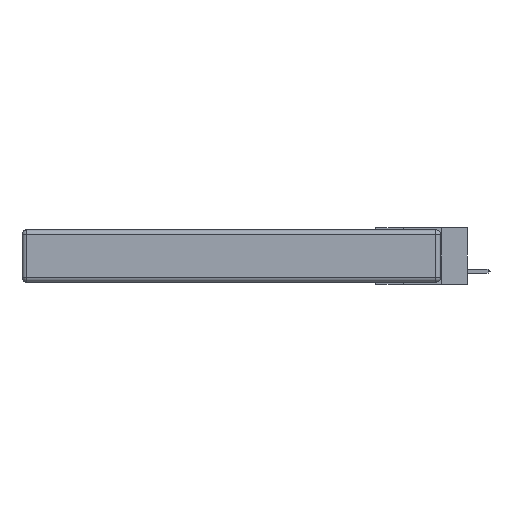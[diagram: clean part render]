
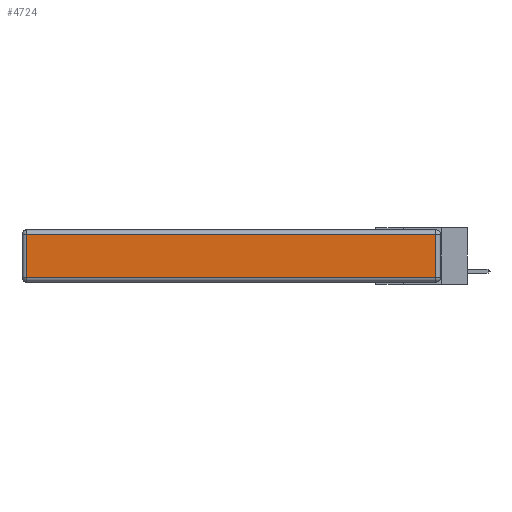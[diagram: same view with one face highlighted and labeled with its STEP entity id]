
A CAD part, left-side view. The second image highlights one B-rep face of the part: STEP entity #4724.
In plain terms, the highlighted planar face has unit normal (-1, 0, 0).
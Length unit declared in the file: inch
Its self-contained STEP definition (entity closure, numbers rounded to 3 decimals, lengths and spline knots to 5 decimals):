
#19 = CARTESIAN_POINT ( 'NONE',  ( 0., 2.72, -0.343 ) ) ;
#664 = CARTESIAN_POINT ( 'NONE',  ( 0., 0., -0.313 ) ) ;
#1249 = DIRECTION ( 'NONE',  ( 0., 0., 1. ) ) ;
#1866 = DIRECTION ( 'NONE',  ( 0., 1., 0. ) ) ;
#1868 = ORIENTED_EDGE ( 'NONE', *, *, #15259, .T. ) ;
#2163 = VERTEX_POINT ( 'NONE', #5978 ) ;
#2335 = CARTESIAN_POINT ( 'NONE',  ( 0., 2.72, -0.03 ) ) ;
#2361 = AXIS2_PLACEMENT_3D ( 'NONE', #16171, #3149, #6937 ) ;
#3149 = DIRECTION ( 'NONE',  ( -1., 0., 0. ) ) ;
#3465 = EDGE_CURVE ( 'NONE', #2163, #12538, #13169, .T. ) ;
#3473 = FACE_OUTER_BOUND ( 'NONE', #11984, .T. ) ;
#3517 = VERTEX_POINT ( 'NONE', #14456 ) ;
#4724 = ADVANCED_FACE ( 'NONE', ( #3473 ), #14804, .T. ) ;
#5080 = VECTOR ( 'NONE', #16360, 39.37008 ) ;
#5199 = ORIENTED_EDGE ( 'NONE', *, *, #8831, .T. ) ;
#5978 = CARTESIAN_POINT ( 'NONE',  ( 0., 0.03, -0.313 ) ) ;
#6816 = VECTOR ( 'NONE', #1866, 39.37008 ) ;
#6937 = DIRECTION ( 'NONE',  ( 0., 0., 1. ) ) ;
#8162 = LINE ( 'NONE', #664, #5080 ) ;
#8401 = CARTESIAN_POINT ( 'NONE',  ( 0., 2.75, -0.03 ) ) ;
#8414 = VERTEX_POINT ( 'NONE', #2335 ) ;
#8831 = EDGE_CURVE ( 'NONE', #12538, #8414, #9465, .T. ) ;
#8909 = ORIENTED_EDGE ( 'NONE', *, *, #3465, .T. ) ;
#9081 = CARTESIAN_POINT ( 'NONE',  ( 0., 0.03, -0.343 ) ) ;
#9465 = LINE ( 'NONE', #8401, #6816 ) ;
#9812 = CARTESIAN_POINT ( 'NONE',  ( 0., 0.03, -0.03 ) ) ;
#10688 = DIRECTION ( 'NONE',  ( 0., 0., -1. ) ) ;
#11320 = VECTOR ( 'NONE', #1249, 39.37008 ) ;
#11984 = EDGE_LOOP ( 'NONE', ( #13062, #8909, #5199, #1868 ) ) ;
#12071 = VECTOR ( 'NONE', #10688, 39.37008 ) ;
#12538 = VERTEX_POINT ( 'NONE', #9812 ) ;
#13062 = ORIENTED_EDGE ( 'NONE', *, *, #16106, .T. ) ;
#13169 = LINE ( 'NONE', #9081, #11320 ) ;
#14456 = CARTESIAN_POINT ( 'NONE',  ( 0., 2.72, -0.313 ) ) ;
#14804 = PLANE ( 'NONE',  #2361 ) ;
#15259 = EDGE_CURVE ( 'NONE', #8414, #3517, #16821, .T. ) ;
#16106 = EDGE_CURVE ( 'NONE', #3517, #2163, #8162, .T. ) ;
#16171 = CARTESIAN_POINT ( 'NONE',  ( 0., 0., -0.343 ) ) ;
#16360 = DIRECTION ( 'NONE',  ( 0., -1., 0. ) ) ;
#16821 = LINE ( 'NONE', #19, #12071 ) ;
